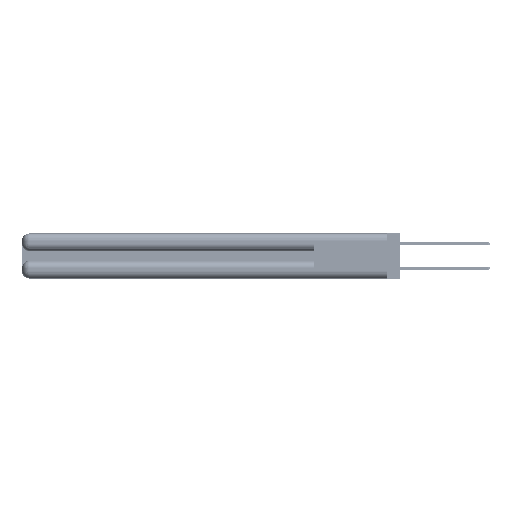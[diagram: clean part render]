
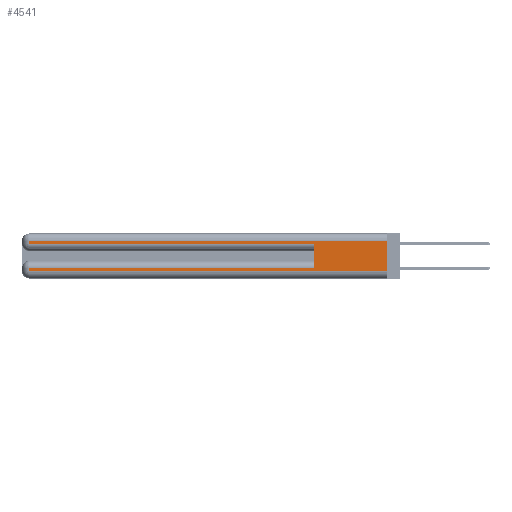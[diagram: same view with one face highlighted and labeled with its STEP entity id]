
A CAD part, left-side view. The second image highlights one B-rep face of the part: STEP entity #4541.
In plain terms, the highlighted planar face has unit normal (-1, 0, 0).
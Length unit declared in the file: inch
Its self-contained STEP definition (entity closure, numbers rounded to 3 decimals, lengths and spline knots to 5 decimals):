
#423 = VECTOR ( 'NONE', #52790, 39.37008 ) ;
#585 = EDGE_CURVE ( 'NONE', #1048, #20874, #35233, .T. ) ;
#930 = CARTESIAN_POINT ( 'NONE',  ( 0., 2.94, 0.31 ) ) ;
#1048 = VERTEX_POINT ( 'NONE', #22752 ) ;
#1496 = CARTESIAN_POINT ( 'NONE',  ( 0., 2.94, 0.37 ) ) ;
#1780 = EDGE_CURVE ( 'NONE', #2805, #27684, #2233, .T. ) ;
#2032 = DIRECTION ( 'NONE',  ( 0., 0., -1. ) ) ;
#2233 = LINE ( 'NONE', #48372, #3529 ) ;
#2331 = LINE ( 'NONE', #18238, #37752 ) ;
#2805 = VERTEX_POINT ( 'NONE', #17704 ) ;
#3250 = LINE ( 'NONE', #1496, #20583 ) ;
#3251 = VERTEX_POINT ( 'NONE', #4023 ) ;
#3399 = EDGE_CURVE ( 'NONE', #2805, #29355, #34235, .T. ) ;
#3529 = VECTOR ( 'NONE', #10976, 39.37008 ) ;
#4023 = CARTESIAN_POINT ( 'NONE',  ( 0., 2.94, 0.06 ) ) ;
#4541 = ADVANCED_FACE ( 'NONE', ( #40688 ), #49010, .F. ) ;
#4945 = CARTESIAN_POINT ( 'NONE',  ( 0., 0., 0.285 ) ) ;
#5865 = DIRECTION ( 'NONE',  ( 0., 1., 0. ) ) ;
#10000 = EDGE_LOOP ( 'NONE', ( #33855, #52073, #19840, #22046, #32903, #16397, #22312, #43484 ) ) ;
#10464 = EDGE_CURVE ( 'NONE', #41109, #20874, #37143, .T. ) ;
#10976 = DIRECTION ( 'NONE',  ( 0., 0., -1. ) ) ;
#11178 = CARTESIAN_POINT ( 'NONE',  ( 0., 0., 0.06 ) ) ;
#13204 = DIRECTION ( 'NONE',  ( 0., -1., 0. ) ) ;
#13213 = CARTESIAN_POINT ( 'NONE',  ( 0., 0., 0.06 ) ) ;
#13334 = VECTOR ( 'NONE', #24524, 39.37008 ) ;
#13759 = EDGE_CURVE ( 'NONE', #1048, #25823, #2331, .T. ) ;
#16397 = ORIENTED_EDGE ( 'NONE', *, *, #13759, .T. ) ;
#16787 = VECTOR ( 'NONE', #50559, 39.37008 ) ;
#17704 = CARTESIAN_POINT ( 'NONE',  ( 0., 0., 0.31 ) ) ;
#18238 = CARTESIAN_POINT ( 'NONE',  ( 0., 0., 0.085 ) ) ;
#18789 = VECTOR ( 'NONE', #33845, 39.37008 ) ;
#19840 = ORIENTED_EDGE ( 'NONE', *, *, #31340, .T. ) ;
#20228 = CARTESIAN_POINT ( 'NONE',  ( 0., 0.6, 0.145 ) ) ;
#20583 = VECTOR ( 'NONE', #2032, 39.37008 ) ;
#20874 = VERTEX_POINT ( 'NONE', #21177 ) ;
#21177 = CARTESIAN_POINT ( 'NONE',  ( 0., 0.6, 0.285 ) ) ;
#22046 = ORIENTED_EDGE ( 'NONE', *, *, #10464, .T. ) ;
#22312 = ORIENTED_EDGE ( 'NONE', *, *, #25176, .T. ) ;
#22752 = CARTESIAN_POINT ( 'NONE',  ( 0., 0.6, 0.085 ) ) ;
#23813 = DIRECTION ( 'NONE',  ( 1., 0., 0. ) ) ;
#24524 = DIRECTION ( 'NONE',  ( 0., 0., 1. ) ) ;
#25176 = EDGE_CURVE ( 'NONE', #25823, #3251, #41018, .T. ) ;
#25549 = VECTOR ( 'NONE', #13204, 39.37008 ) ;
#25823 = VERTEX_POINT ( 'NONE', #45381 ) ;
#27684 = VERTEX_POINT ( 'NONE', #11178 ) ;
#29355 = VERTEX_POINT ( 'NONE', #930 ) ;
#29613 = LINE ( 'NONE', #13213, #16787 ) ;
#31340 = EDGE_CURVE ( 'NONE', #29355, #41109, #3250, .T. ) ;
#32903 = ORIENTED_EDGE ( 'NONE', *, *, #585, .F. ) ;
#33845 = DIRECTION ( 'NONE',  ( 0., 1., 0. ) ) ;
#33855 = ORIENTED_EDGE ( 'NONE', *, *, #1780, .F. ) ;
#34235 = LINE ( 'NONE', #37641, #18789 ) ;
#35233 = LINE ( 'NONE', #20228, #13334 ) ;
#37143 = LINE ( 'NONE', #4945, #25549 ) ;
#37641 = CARTESIAN_POINT ( 'NONE',  ( 0., 0., 0.31 ) ) ;
#37752 = VECTOR ( 'NONE', #5865, 39.37008 ) ;
#40615 = DIRECTION ( 'NONE',  ( 0., 0., -1. ) ) ;
#40688 = FACE_OUTER_BOUND ( 'NONE', #10000, .T. ) ;
#40960 = CARTESIAN_POINT ( 'NONE',  ( 0., 2.94, 0.37 ) ) ;
#41018 = LINE ( 'NONE', #40960, #423 ) ;
#41109 = VERTEX_POINT ( 'NONE', #47021 ) ;
#43484 = ORIENTED_EDGE ( 'NONE', *, *, #47241, .T. ) ;
#45381 = CARTESIAN_POINT ( 'NONE',  ( 0., 2.94, 0.085 ) ) ;
#46342 = AXIS2_PLACEMENT_3D ( 'NONE', #52973, #23813, #40615 ) ;
#47021 = CARTESIAN_POINT ( 'NONE',  ( 0., 2.94, 0.285 ) ) ;
#47241 = EDGE_CURVE ( 'NONE', #3251, #27684, #29613, .T. ) ;
#48372 = CARTESIAN_POINT ( 'NONE',  ( 0., 0., 0.37 ) ) ;
#49010 = PLANE ( 'NONE',  #46342 ) ;
#50559 = DIRECTION ( 'NONE',  ( 0., -1., 0. ) ) ;
#52073 = ORIENTED_EDGE ( 'NONE', *, *, #3399, .T. ) ;
#52790 = DIRECTION ( 'NONE',  ( 0., 0., -1. ) ) ;
#52973 = CARTESIAN_POINT ( 'NONE',  ( 0., 0., 0.37 ) ) ;
